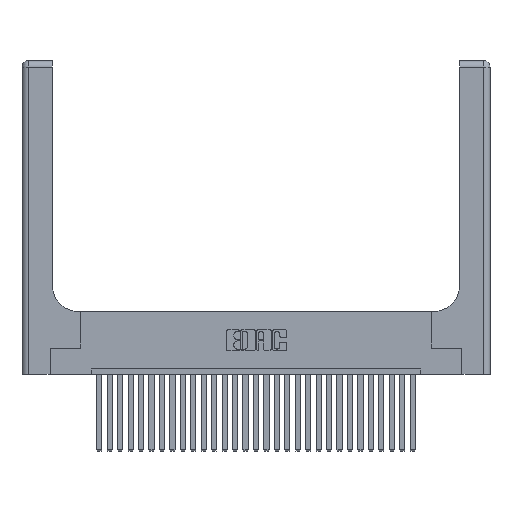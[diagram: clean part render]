
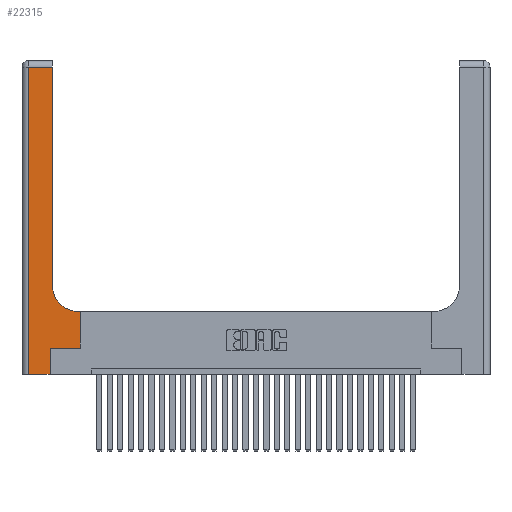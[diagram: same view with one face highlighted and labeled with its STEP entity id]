
A CAD part, top view. The second image highlights one B-rep face of the part: STEP entity #22315.
In plain terms, the highlighted planar face has unit normal (0, 0, 1).
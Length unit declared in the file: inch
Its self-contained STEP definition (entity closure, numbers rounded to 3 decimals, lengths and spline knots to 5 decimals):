
#89 = ORIENTED_EDGE ( 'NONE', *, *, #12667, .T. ) ;
#132 = DIRECTION ( 'NONE',  ( 1., 0., 0. ) ) ;
#408 = LINE ( 'NONE', #19837, #23525 ) ;
#899 = AXIS2_PLACEMENT_3D ( 'NONE', #9028, #13658, #132 ) ;
#1362 = VERTEX_POINT ( 'NONE', #12647 ) ;
#2119 = DIRECTION ( 'NONE',  ( 0., 1., 0. ) ) ;
#2844 = LINE ( 'NONE', #4347, #26291 ) ;
#3406 = DIRECTION ( 'NONE',  ( 1., 0., 0. ) ) ;
#3865 = ORIENTED_EDGE ( 'NONE', *, *, #28362, .T. ) ;
#4347 = CARTESIAN_POINT ( 'NONE',  ( 0.06, 3., 0.37 ) ) ;
#4954 = VERTEX_POINT ( 'NONE', #26954 ) ;
#5474 = DIRECTION ( 'NONE',  ( 0., 0., -1. ) ) ;
#5775 = CARTESIAN_POINT ( 'NONE',  ( 0.269, 0.25, 0.37 ) ) ;
#6097 = FACE_OUTER_BOUND ( 'NONE', #18123, .T. ) ;
#6435 = CARTESIAN_POINT ( 'NONE',  ( 0.5585, 0.25, 0.37 ) ) ;
#6523 = LINE ( 'NONE', #24414, #28825 ) ;
#6678 = DIRECTION ( 'NONE',  ( 0., -1., 0. ) ) ;
#7517 = LINE ( 'NONE', #17967, #15089 ) ;
#7911 = CARTESIAN_POINT ( 'NONE',  ( 0.5585, 0.6, 0.37 ) ) ;
#8506 = VERTEX_POINT ( 'NONE', #9117 ) ;
#8739 = CARTESIAN_POINT ( 'NONE',  ( 0.269, 0., 0.37 ) ) ;
#9028 = CARTESIAN_POINT ( 'NONE',  ( 0.5415, 0.85, 0.37 ) ) ;
#9045 = EDGE_CURVE ( 'NONE', #19544, #4954, #9701, .T. ) ;
#9117 = CARTESIAN_POINT ( 'NONE',  ( 0.2915, 2.94, 0.37 ) ) ;
#9210 = ORIENTED_EDGE ( 'NONE', *, *, #9045, .T. ) ;
#9701 = CIRCLE ( 'NONE', #899, 0.25 ) ;
#10143 = VECTOR ( 'NONE', #20942, 39.37008 ) ;
#10350 = EDGE_CURVE ( 'NONE', #17786, #29215, #7517, .T. ) ;
#10579 = VERTEX_POINT ( 'NONE', #6435 ) ;
#10821 = ORIENTED_EDGE ( 'NONE', *, *, #21054, .T. ) ;
#12647 = CARTESIAN_POINT ( 'NONE',  ( 0.06, 2.94, 0.37 ) ) ;
#12667 = EDGE_CURVE ( 'NONE', #8506, #1362, #16760, .T. ) ;
#13600 = CARTESIAN_POINT ( 'NONE',  ( 0., 0., 0.37 ) ) ;
#13658 = DIRECTION ( 'NONE',  ( 0., 0., -1. ) ) ;
#13850 = VECTOR ( 'NONE', #21773, 39.37008 ) ;
#14482 = CARTESIAN_POINT ( 'NONE',  ( 0., 2.94, 0.37 ) ) ;
#14538 = CARTESIAN_POINT ( 'NONE',  ( 0., 3., 0.37 ) ) ;
#15089 = VECTOR ( 'NONE', #2119, 39.37008 ) ;
#15195 = DIRECTION ( 'NONE',  ( 0., 1., 0. ) ) ;
#15356 = VECTOR ( 'NONE', #20540, 39.37008 ) ;
#15686 = EDGE_CURVE ( 'NONE', #1362, #21667, #2844, .T. ) ;
#16760 = LINE ( 'NONE', #14482, #13850 ) ;
#17672 = VERTEX_POINT ( 'NONE', #7911 ) ;
#17786 = VERTEX_POINT ( 'NONE', #8739 ) ;
#17869 = EDGE_CURVE ( 'NONE', #29215, #10579, #27982, .T. ) ;
#17967 = CARTESIAN_POINT ( 'NONE',  ( 0.269, 0., 0.37 ) ) ;
#18123 = EDGE_LOOP ( 'NONE', ( #28368, #89, #23128, #24286, #26656, #20827, #3865, #10821, #9210 ) ) ;
#18136 = CARTESIAN_POINT ( 'NONE',  ( 0.5585, 0.25, 0.37 ) ) ;
#18181 = LINE ( 'NONE', #13600, #19238 ) ;
#18811 = DIRECTION ( 'NONE',  ( -1., 0., 0. ) ) ;
#19238 = VECTOR ( 'NONE', #3406, 39.37008 ) ;
#19388 = EDGE_CURVE ( 'NONE', #21667, #17786, #18181, .T. ) ;
#19544 = VERTEX_POINT ( 'NONE', #25292 ) ;
#19837 = CARTESIAN_POINT ( 'NONE',  ( 0.2915, 3., 0.37 ) ) ;
#20540 = DIRECTION ( 'NONE',  ( 1., 0., 0. ) ) ;
#20645 = CARTESIAN_POINT ( 'NONE',  ( 0.269, 0.25, 0.37 ) ) ;
#20827 = ORIENTED_EDGE ( 'NONE', *, *, #17869, .T. ) ;
#20942 = DIRECTION ( 'NONE',  ( 0., 1., 0. ) ) ;
#21054 = EDGE_CURVE ( 'NONE', #17672, #19544, #6523, .T. ) ;
#21430 = PLANE ( 'NONE',  #26706 ) ;
#21667 = VERTEX_POINT ( 'NONE', #25577 ) ;
#21773 = DIRECTION ( 'NONE',  ( -1., 0., 0. ) ) ;
#22315 = ADVANCED_FACE ( 'NONE', ( #6097 ), #21430, .F. ) ;
#23128 = ORIENTED_EDGE ( 'NONE', *, *, #15686, .T. ) ;
#23525 = VECTOR ( 'NONE', #15195, 39.37008 ) ;
#24142 = DIRECTION ( 'NONE',  ( -1., 0., 0. ) ) ;
#24286 = ORIENTED_EDGE ( 'NONE', *, *, #19388, .T. ) ;
#24414 = CARTESIAN_POINT ( 'NONE',  ( 0.2915, 0.6, 0.37 ) ) ;
#25292 = CARTESIAN_POINT ( 'NONE',  ( 0.5415, 0.6, 0.37 ) ) ;
#25577 = CARTESIAN_POINT ( 'NONE',  ( 0.06, 0., 0.37 ) ) ;
#26022 = LINE ( 'NONE', #18136, #10143 ) ;
#26291 = VECTOR ( 'NONE', #6678, 39.37008 ) ;
#26656 = ORIENTED_EDGE ( 'NONE', *, *, #10350, .T. ) ;
#26706 = AXIS2_PLACEMENT_3D ( 'NONE', #14538, #5474, #24142 ) ;
#26954 = CARTESIAN_POINT ( 'NONE',  ( 0.2915, 0.85, 0.37 ) ) ;
#27982 = LINE ( 'NONE', #20645, #15356 ) ;
#28018 = EDGE_CURVE ( 'NONE', #4954, #8506, #408, .T. ) ;
#28362 = EDGE_CURVE ( 'NONE', #10579, #17672, #26022, .T. ) ;
#28368 = ORIENTED_EDGE ( 'NONE', *, *, #28018, .T. ) ;
#28825 = VECTOR ( 'NONE', #18811, 39.37008 ) ;
#29215 = VERTEX_POINT ( 'NONE', #5775 ) ;
